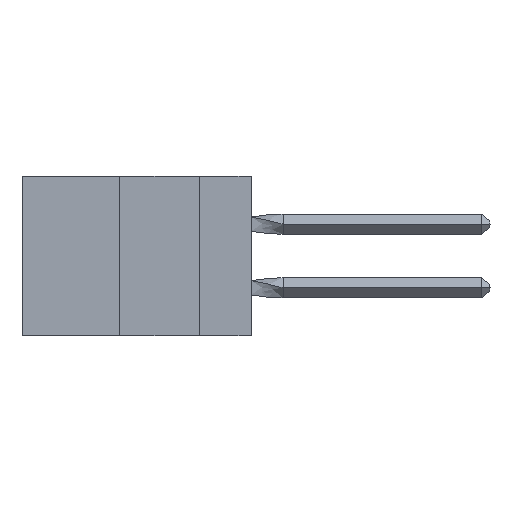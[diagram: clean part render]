
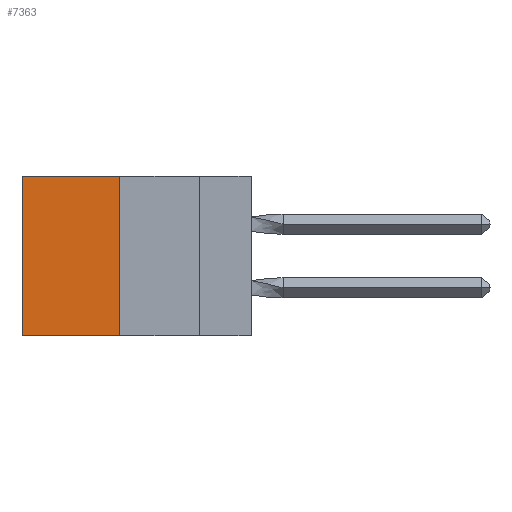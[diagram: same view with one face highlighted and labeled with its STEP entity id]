
A CAD part, left-side view. The second image highlights one B-rep face of the part: STEP entity #7363.
In plain terms, the highlighted planar face has unit normal (-1, 0, 0).
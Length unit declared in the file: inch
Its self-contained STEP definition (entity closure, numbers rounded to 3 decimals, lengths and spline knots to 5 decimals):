
#346 = CARTESIAN_POINT ( 'NONE',  ( 0.305, 0.413, 0. ) ) ;
#710 = EDGE_LOOP ( 'NONE', ( #11955, #2548, #15690, #13627 ) ) ;
#774 = EDGE_CURVE ( 'NONE', #20433, #1730, #14843, .T. ) ;
#1518 = VERTEX_POINT ( 'NONE', #15601 ) ;
#1634 = DIRECTION ( 'NONE',  ( 1., 0., 0. ) ) ;
#1730 = VERTEX_POINT ( 'NONE', #4025 ) ;
#2163 = AXIS2_PLACEMENT_3D ( 'NONE', #13789, #1634, #3245 ) ;
#2548 = ORIENTED_EDGE ( 'NONE', *, *, #17246, .F. ) ;
#3244 = CARTESIAN_POINT ( 'NONE',  ( 0.305, 0.72, 0. ) ) ;
#3245 = DIRECTION ( 'NONE',  ( 0., 0., -1. ) ) ;
#3698 = VECTOR ( 'NONE', #10635, 39.37008 ) ;
#4025 = CARTESIAN_POINT ( 'NONE',  ( 0.305, 0.72, -0.5 ) ) ;
#5638 = LINE ( 'NONE', #10313, #13090 ) ;
#6372 = VECTOR ( 'NONE', #9052, 39.37008 ) ;
#6575 = VECTOR ( 'NONE', #8093, 39.37008 ) ;
#7363 = ADVANCED_FACE ( 'NONE', ( #13748 ), #21060, .F. ) ;
#8093 = DIRECTION ( 'NONE',  ( 0., 0., -1. ) ) ;
#8395 = LINE ( 'NONE', #19436, #3698 ) ;
#9052 = DIRECTION ( 'NONE',  ( 0., 1., 0. ) ) ;
#9203 = VERTEX_POINT ( 'NONE', #13233 ) ;
#10139 = DIRECTION ( 'NONE',  ( 0., 1., 0. ) ) ;
#10313 = CARTESIAN_POINT ( 'NONE',  ( 0.305, 0.413, -0.5 ) ) ;
#10635 = DIRECTION ( 'NONE',  ( 0., 0., -1. ) ) ;
#11955 = ORIENTED_EDGE ( 'NONE', *, *, #774, .T. ) ;
#13090 = VECTOR ( 'NONE', #10139, 39.37008 ) ;
#13233 = CARTESIAN_POINT ( 'NONE',  ( 0.305, 0.413, -0.5 ) ) ;
#13237 = EDGE_CURVE ( 'NONE', #1518, #9203, #8395, .T. ) ;
#13462 = CARTESIAN_POINT ( 'NONE',  ( 0.305, 0.72, -0.5 ) ) ;
#13627 = ORIENTED_EDGE ( 'NONE', *, *, #18712, .T. ) ;
#13748 = FACE_OUTER_BOUND ( 'NONE', #710, .T. ) ;
#13789 = CARTESIAN_POINT ( 'NONE',  ( 0.305, 0.413, -0.5 ) ) ;
#14843 = LINE ( 'NONE', #13462, #6575 ) ;
#15601 = CARTESIAN_POINT ( 'NONE',  ( 0.305, 0.413, 0. ) ) ;
#15690 = ORIENTED_EDGE ( 'NONE', *, *, #13237, .F. ) ;
#16038 = LINE ( 'NONE', #346, #6372 ) ;
#17246 = EDGE_CURVE ( 'NONE', #9203, #1730, #5638, .T. ) ;
#18712 = EDGE_CURVE ( 'NONE', #1518, #20433, #16038, .T. ) ;
#19436 = CARTESIAN_POINT ( 'NONE',  ( 0.305, 0.413, -0.5 ) ) ;
#20433 = VERTEX_POINT ( 'NONE', #3244 ) ;
#21060 = PLANE ( 'NONE',  #2163 ) ;
